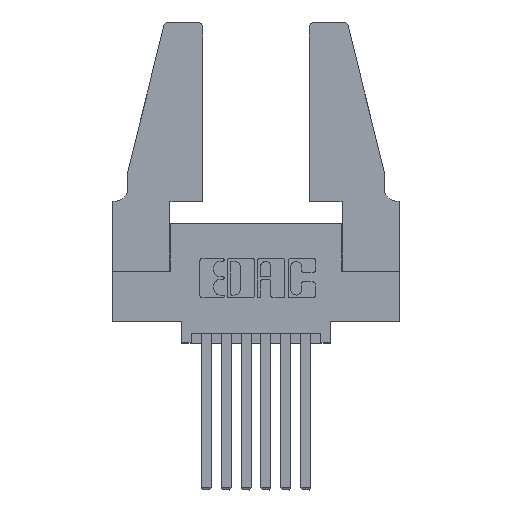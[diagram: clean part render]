
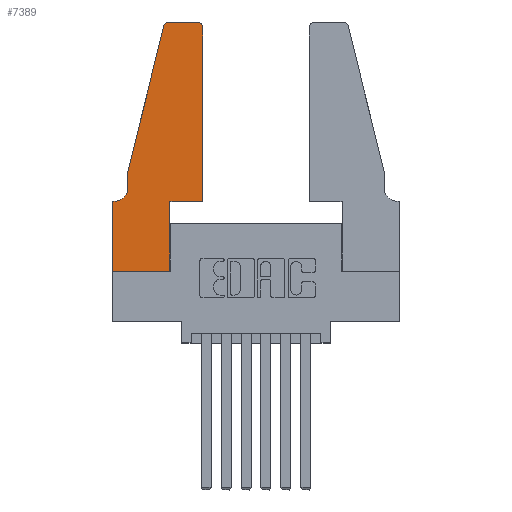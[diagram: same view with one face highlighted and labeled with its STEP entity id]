
A CAD part, top view. The second image highlights one B-rep face of the part: STEP entity #7389.
In plain terms, the highlighted planar face has unit normal (0, 0, 1).
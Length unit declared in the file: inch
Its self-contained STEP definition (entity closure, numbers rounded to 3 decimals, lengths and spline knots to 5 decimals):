
#34 = VECTOR ( 'NONE', #9500, 39.37008 ) ;
#337 = CARTESIAN_POINT ( 'NONE',  ( 0.0755, 0.42, 0.37 ) ) ;
#362 = AXIS2_PLACEMENT_3D ( 'NONE', #3548, #10689, #5392 ) ;
#509 = CARTESIAN_POINT ( 'NONE',  ( 0.4505, 0.35, 0.37 ) ) ;
#532 = DIRECTION ( 'NONE',  ( 0., 1., 0. ) ) ;
#646 = VERTEX_POINT ( 'NONE', #9066 ) ;
#808 = DIRECTION ( 'NONE',  ( -1., 0., 0. ) ) ;
#927 = DIRECTION ( 'NONE',  ( 0., 0., 1. ) ) ;
#1243 = EDGE_CURVE ( 'NONE', #11419, #1875, #11331, .T. ) ;
#1254 = CARTESIAN_POINT ( 'NONE',  ( 0., 0., 0.37 ) ) ;
#1342 = ORIENTED_EDGE ( 'NONE', *, *, #2374, .T. ) ;
#1379 = LINE ( 'NONE', #5990, #8383 ) ;
#1467 = CARTESIAN_POINT ( 'NONE',  ( 0.4505, 1.22, 0.37 ) ) ;
#1476 = CARTESIAN_POINT ( 'NONE',  ( 0.4505, 0.35, 0.37 ) ) ;
#1868 = EDGE_CURVE ( 'NONE', #9388, #3879, #8664, .T. ) ;
#1875 = VERTEX_POINT ( 'NONE', #1467 ) ;
#1907 = DIRECTION ( 'NONE',  ( 1., 0., 0. ) ) ;
#2077 = CARTESIAN_POINT ( 'NONE',  ( 0.0755, 0.35, 0.37 ) ) ;
#2256 = CARTESIAN_POINT ( 'NONE',  ( 0.2865, 0.35, 0.37 ) ) ;
#2341 = AXIS2_PLACEMENT_3D ( 'NONE', #9158, #3759, #10023 ) ;
#2374 = EDGE_CURVE ( 'NONE', #3879, #646, #3266, .T. ) ;
#2680 = VECTOR ( 'NONE', #1907, 39.37008 ) ;
#2699 = VERTEX_POINT ( 'NONE', #337 ) ;
#2929 = CARTESIAN_POINT ( 'NONE',  ( 0., 0., 0.37 ) ) ;
#2932 = VECTOR ( 'NONE', #808, 39.37008 ) ;
#2942 = ORIENTED_EDGE ( 'NONE', *, *, #6794, .T. ) ;
#2986 = CARTESIAN_POINT ( 'NONE',  ( 0.2865, 0.35, 0.37 ) ) ;
#3266 = LINE ( 'NONE', #3988, #2680 ) ;
#3503 = AXIS2_PLACEMENT_3D ( 'NONE', #9628, #4255, #10491 ) ;
#3510 = VERTEX_POINT ( 'NONE', #7171 ) ;
#3548 = CARTESIAN_POINT ( 'NONE',  ( 0., 0.35, 0.37 ) ) ;
#3564 = CARTESIAN_POINT ( 'NONE',  ( 0.25487, 1.22718, 0.37 ) ) ;
#3641 = ORIENTED_EDGE ( 'NONE', *, *, #7669, .T. ) ;
#3678 = ORIENTED_EDGE ( 'NONE', *, *, #8945, .T. ) ;
#3759 = DIRECTION ( 'NONE',  ( 0., 0., 1. ) ) ;
#3879 = VERTEX_POINT ( 'NONE', #1254 ) ;
#3988 = CARTESIAN_POINT ( 'NONE',  ( 0., 0., 0.37 ) ) ;
#4184 = EDGE_CURVE ( 'NONE', #9155, #7232, #5355, .T. ) ;
#4255 = DIRECTION ( 'NONE',  ( 0., 0., -1. ) ) ;
#4464 = PLANE ( 'NONE',  #362 ) ;
#4469 = CARTESIAN_POINT ( 'NONE',  ( 0.2605, 1.25, 0.37 ) ) ;
#4553 = ORIENTED_EDGE ( 'NONE', *, *, #10356, .T. ) ;
#4713 = VECTOR ( 'NONE', #4849, 39.37008 ) ;
#4837 = VECTOR ( 'NONE', #532, 39.37008 ) ;
#4849 = DIRECTION ( 'NONE',  ( 0., -1., 0. ) ) ;
#4985 = DIRECTION ( 'NONE',  ( -0.239, -0.971, 0. ) ) ;
#5115 = DIRECTION ( 'NONE',  ( 0., -1., 0. ) ) ;
#5183 = CARTESIAN_POINT ( 'NONE',  ( 0.284, 1.25, 0.37 ) ) ;
#5355 = LINE ( 'NONE', #4469, #2932 ) ;
#5392 = DIRECTION ( 'NONE',  ( 1., 0., 0. ) ) ;
#5420 = CARTESIAN_POINT ( 'NONE',  ( 0., 0.35, 0.37 ) ) ;
#5990 = CARTESIAN_POINT ( 'NONE',  ( 0.0755, 0.5, 0.37 ) ) ;
#6098 = ORIENTED_EDGE ( 'NONE', *, *, #10530, .T. ) ;
#6448 = CARTESIAN_POINT ( 'NONE',  ( 0.4205, 1.22, 0.37 ) ) ;
#6556 = VECTOR ( 'NONE', #5115, 39.37008 ) ;
#6696 = VECTOR ( 'NONE', #8929, 39.37008 ) ;
#6719 = VECTOR ( 'NONE', #9330, 39.37008 ) ;
#6794 = EDGE_CURVE ( 'NONE', #1875, #9155, #10961, .T. ) ;
#7114 = ORIENTED_EDGE ( 'NONE', *, *, #1243, .T. ) ;
#7166 = ORIENTED_EDGE ( 'NONE', *, *, #9599, .T. ) ;
#7171 = CARTESIAN_POINT ( 'NONE',  ( 0.0755, 0.5, 0.37 ) ) ;
#7232 = VERTEX_POINT ( 'NONE', #5183 ) ;
#7247 = EDGE_LOOP ( 'NONE', ( #9868, #3678, #4553, #3641, #8786, #7166, #10055, #1342, #10476, #6098, #7114, #2942 ) ) ;
#7354 = DIRECTION ( 'NONE',  ( 1., 0., 0. ) ) ;
#7389 = ADVANCED_FACE ( 'NONE', ( #9897 ), #4464, .T. ) ;
#7497 = CARTESIAN_POINT ( 'NONE',  ( 0.0055, 0.35, 0.37 ) ) ;
#7592 = VERTEX_POINT ( 'NONE', #7497 ) ;
#7669 = EDGE_CURVE ( 'NONE', #3510, #2699, #9494, .T. ) ;
#8311 = VERTEX_POINT ( 'NONE', #2986 ) ;
#8383 = VECTOR ( 'NONE', #4985, 39.37008 ) ;
#8664 = LINE ( 'NONE', #2929, #6556 ) ;
#8786 = ORIENTED_EDGE ( 'NONE', *, *, #9794, .T. ) ;
#8929 = DIRECTION ( 'NONE',  ( 1., 0., 0. ) ) ;
#8945 = EDGE_CURVE ( 'NONE', #7232, #9987, #11222, .T. ) ;
#9002 = AXIS2_PLACEMENT_3D ( 'NONE', #6448, #927, #7354 ) ;
#9066 = CARTESIAN_POINT ( 'NONE',  ( 0.2865, 0., 0.37 ) ) ;
#9081 = LINE ( 'NONE', #2077, #6719 ) ;
#9155 = VERTEX_POINT ( 'NONE', #10240 ) ;
#9158 = CARTESIAN_POINT ( 'NONE',  ( 0.284, 1.22, 0.37 ) ) ;
#9330 = DIRECTION ( 'NONE',  ( -1., 0., 0. ) ) ;
#9388 = VERTEX_POINT ( 'NONE', #5420 ) ;
#9494 = LINE ( 'NONE', #11040, #4713 ) ;
#9500 = DIRECTION ( 'NONE',  ( 0., 1., 0. ) ) ;
#9599 = EDGE_CURVE ( 'NONE', #7592, #9388, #9081, .T. ) ;
#9628 = CARTESIAN_POINT ( 'NONE',  ( 0.0055, 0.42, 0.37 ) ) ;
#9742 = LINE ( 'NONE', #2256, #34 ) ;
#9754 = CIRCLE ( 'NONE', #3503, 0.07 ) ;
#9794 = EDGE_CURVE ( 'NONE', #2699, #7592, #9754, .T. ) ;
#9868 = ORIENTED_EDGE ( 'NONE', *, *, #4184, .T. ) ;
#9897 = FACE_OUTER_BOUND ( 'NONE', #7247, .T. ) ;
#9987 = VERTEX_POINT ( 'NONE', #3564 ) ;
#10023 = DIRECTION ( 'NONE',  ( 1., 0., 0. ) ) ;
#10055 = ORIENTED_EDGE ( 'NONE', *, *, #1868, .T. ) ;
#10240 = CARTESIAN_POINT ( 'NONE',  ( 0.4205, 1.25, 0.37 ) ) ;
#10356 = EDGE_CURVE ( 'NONE', #9987, #3510, #1379, .T. ) ;
#10476 = ORIENTED_EDGE ( 'NONE', *, *, #10943, .T. ) ;
#10491 = DIRECTION ( 'NONE',  ( -1., 0., 0. ) ) ;
#10530 = EDGE_CURVE ( 'NONE', #8311, #11419, #11315, .T. ) ;
#10615 = CARTESIAN_POINT ( 'NONE',  ( 0.4505, 0.35, 0.37 ) ) ;
#10689 = DIRECTION ( 'NONE',  ( 0., 0., 1. ) ) ;
#10943 = EDGE_CURVE ( 'NONE', #646, #8311, #9742, .T. ) ;
#10961 = CIRCLE ( 'NONE', #9002, 0.03 ) ;
#11040 = CARTESIAN_POINT ( 'NONE',  ( 0.0755, 0.5, 0.37 ) ) ;
#11222 = CIRCLE ( 'NONE', #2341, 0.03 ) ;
#11315 = LINE ( 'NONE', #10615, #6696 ) ;
#11331 = LINE ( 'NONE', #509, #4837 ) ;
#11419 = VERTEX_POINT ( 'NONE', #1476 ) ;
